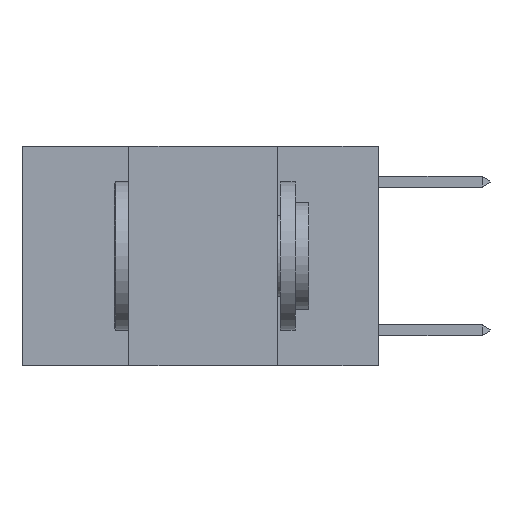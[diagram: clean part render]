
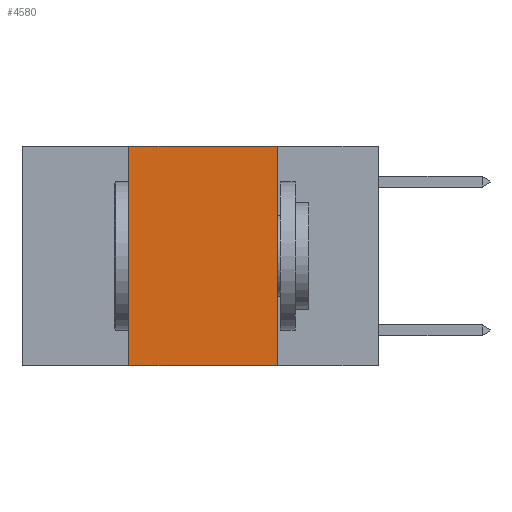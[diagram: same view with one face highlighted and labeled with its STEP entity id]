
A CAD part, left-side view. The second image highlights one B-rep face of the part: STEP entity #4580.
In plain terms, the highlighted planar face has unit normal (-1, 0, 0).
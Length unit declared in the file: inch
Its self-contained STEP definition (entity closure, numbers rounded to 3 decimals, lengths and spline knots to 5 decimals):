
#71 = EDGE_CURVE ( 'NONE', #1941, #6560, #10913, .T. ) ;
#394 = VERTEX_POINT ( 'NONE', #18752 ) ;
#1843 = EDGE_CURVE ( 'NONE', #6156, #6560, #14495, .T. ) ;
#1941 = VERTEX_POINT ( 'NONE', #19379 ) ;
#3033 = DIRECTION ( 'NONE',  ( 0., 0., 1. ) ) ;
#3948 = VECTOR ( 'NONE', #16477, 39.37008 ) ;
#4003 = FACE_OUTER_BOUND ( 'NONE', #14656, .T. ) ;
#4186 = EDGE_CURVE ( 'NONE', #394, #6156, #6344, .T. ) ;
#4580 = ADVANCED_FACE ( 'NONE', ( #4003 ), #12588, .F. ) ;
#4787 = VECTOR ( 'NONE', #6149, 39.37008 ) ;
#5940 = ORIENTED_EDGE ( 'NONE', *, *, #4186, .F. ) ;
#6149 = DIRECTION ( 'NONE',  ( 0., 0., -1. ) ) ;
#6156 = VERTEX_POINT ( 'NONE', #25334 ) ;
#6283 = CARTESIAN_POINT ( 'NONE',  ( 0., 0.6, 0. ) ) ;
#6344 = LINE ( 'NONE', #9994, #3948 ) ;
#6560 = VERTEX_POINT ( 'NONE', #15035 ) ;
#7229 = LINE ( 'NONE', #21549, #19285 ) ;
#9260 = ORIENTED_EDGE ( 'NONE', *, *, #71, .T. ) ;
#9980 = AXIS2_PLACEMENT_3D ( 'NONE', #6283, #18975, #20995 ) ;
#9994 = CARTESIAN_POINT ( 'NONE',  ( 0., 0.6, 0. ) ) ;
#10913 = LINE ( 'NONE', #11045, #18946 ) ;
#11045 = CARTESIAN_POINT ( 'NONE',  ( 0., 0.6, -0.37 ) ) ;
#12588 = PLANE ( 'NONE',  #9980 ) ;
#12872 = ORIENTED_EDGE ( 'NONE', *, *, #1843, .F. ) ;
#14495 = LINE ( 'NONE', #24513, #4787 ) ;
#14656 = EDGE_LOOP ( 'NONE', ( #12872, #5940, #18678, #9260 ) ) ;
#15035 = CARTESIAN_POINT ( 'NONE',  ( 0., 0.17, -0.37 ) ) ;
#16477 = DIRECTION ( 'NONE',  ( 0., -1., 0. ) ) ;
#17569 = EDGE_CURVE ( 'NONE', #1941, #394, #7229, .T. ) ;
#18678 = ORIENTED_EDGE ( 'NONE', *, *, #17569, .F. ) ;
#18752 = CARTESIAN_POINT ( 'NONE',  ( 0., 0.42, 0. ) ) ;
#18946 = VECTOR ( 'NONE', #25246, 39.37008 ) ;
#18975 = DIRECTION ( 'NONE',  ( 1., 0., 0. ) ) ;
#19285 = VECTOR ( 'NONE', #3033, 39.37008 ) ;
#19379 = CARTESIAN_POINT ( 'NONE',  ( 0., 0.42, -0.37 ) ) ;
#20995 = DIRECTION ( 'NONE',  ( 0., 0., -1. ) ) ;
#21549 = CARTESIAN_POINT ( 'NONE',  ( 0., 0.42, 0. ) ) ;
#24513 = CARTESIAN_POINT ( 'NONE',  ( 0., 0.17, 0. ) ) ;
#25246 = DIRECTION ( 'NONE',  ( 0., -1., 0. ) ) ;
#25334 = CARTESIAN_POINT ( 'NONE',  ( 0., 0.17, 0. ) ) ;
